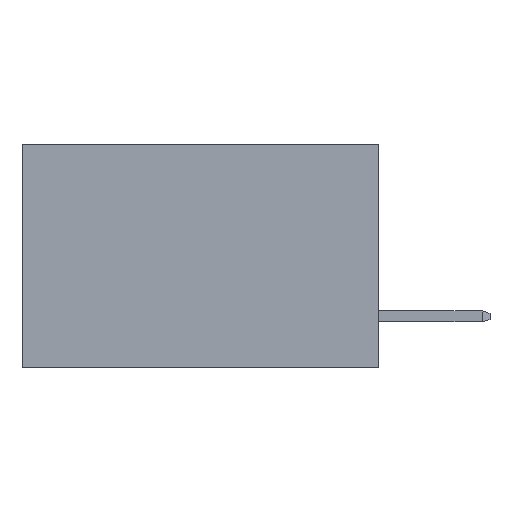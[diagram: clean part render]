
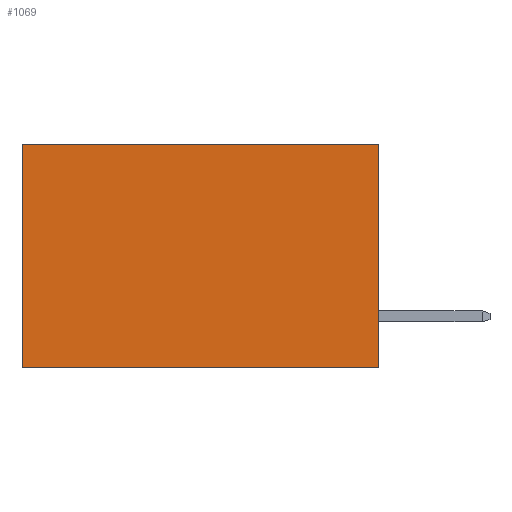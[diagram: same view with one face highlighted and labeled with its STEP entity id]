
A CAD part, left-side view. The second image highlights one B-rep face of the part: STEP entity #1069.
In plain terms, the highlighted planar face has unit normal (-1, 0, 0).
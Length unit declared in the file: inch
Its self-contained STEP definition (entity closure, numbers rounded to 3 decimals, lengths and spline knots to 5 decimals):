
#122 = CARTESIAN_POINT ( 'NONE',  ( 0.277, 0.59, 0. ) ) ;
#636 = LINE ( 'NONE', #6959, #4167 ) ;
#1069 = ADVANCED_FACE ( 'NONE', ( #4967 ), #3012, .F. ) ;
#1996 = EDGE_CURVE ( 'NONE', #3970, #4097, #5149, .T. ) ;
#2041 = DIRECTION ( 'NONE',  ( 0., 1., 0. ) ) ;
#2179 = ORIENTED_EDGE ( 'NONE', *, *, #1996, .T. ) ;
#2214 = ORIENTED_EDGE ( 'NONE', *, *, #4789, .F. ) ;
#2226 = ORIENTED_EDGE ( 'NONE', *, *, #6334, .F. ) ;
#2277 = ORIENTED_EDGE ( 'NONE', *, *, #4604, .T. ) ;
#2321 = VERTEX_POINT ( 'NONE', #3637 ) ;
#2394 = CARTESIAN_POINT ( 'NONE',  ( 0.277, 0.59, -0.37 ) ) ;
#2757 = CARTESIAN_POINT ( 'NONE',  ( 0.277, 0., -0.37 ) ) ;
#3012 = PLANE ( 'NONE',  #5063 ) ;
#3256 = DIRECTION ( 'NONE',  ( 0., 0., -1. ) ) ;
#3299 = DIRECTION ( 'NONE',  ( 1., 0., 0. ) ) ;
#3528 = VECTOR ( 'NONE', #3711, 39.37008 ) ;
#3637 = CARTESIAN_POINT ( 'NONE',  ( 0.277, 0., -0.37 ) ) ;
#3711 = DIRECTION ( 'NONE',  ( 0., 0., -1. ) ) ;
#3881 = CARTESIAN_POINT ( 'NONE',  ( 0.277, 0., 0. ) ) ;
#3970 = VERTEX_POINT ( 'NONE', #122 ) ;
#4097 = VERTEX_POINT ( 'NONE', #6408 ) ;
#4167 = VECTOR ( 'NONE', #7344, 39.37008 ) ;
#4475 = VECTOR ( 'NONE', #2041, 39.37008 ) ;
#4604 = EDGE_CURVE ( 'NONE', #4821, #3970, #7666, .T. ) ;
#4762 = LINE ( 'NONE', #7723, #7584 ) ;
#4789 = EDGE_CURVE ( 'NONE', #2321, #4097, #4762, .T. ) ;
#4821 = VERTEX_POINT ( 'NONE', #5990 ) ;
#4967 = FACE_OUTER_BOUND ( 'NONE', #5997, .T. ) ;
#5063 = AXIS2_PLACEMENT_3D ( 'NONE', #2757, #3299, #3256 ) ;
#5149 = LINE ( 'NONE', #2394, #3528 ) ;
#5990 = CARTESIAN_POINT ( 'NONE',  ( 0.277, 0., 0. ) ) ;
#5997 = EDGE_LOOP ( 'NONE', ( #2179, #2214, #2226, #2277 ) ) ;
#6334 = EDGE_CURVE ( 'NONE', #4821, #2321, #636, .T. ) ;
#6408 = CARTESIAN_POINT ( 'NONE',  ( 0.277, 0.59, -0.37 ) ) ;
#6701 = DIRECTION ( 'NONE',  ( 0., 1., 0. ) ) ;
#6959 = CARTESIAN_POINT ( 'NONE',  ( 0.277, 0., -0.37 ) ) ;
#7344 = DIRECTION ( 'NONE',  ( 0., 0., -1. ) ) ;
#7584 = VECTOR ( 'NONE', #6701, 39.37008 ) ;
#7666 = LINE ( 'NONE', #3881, #4475 ) ;
#7723 = CARTESIAN_POINT ( 'NONE',  ( 0.277, 0., -0.37 ) ) ;
